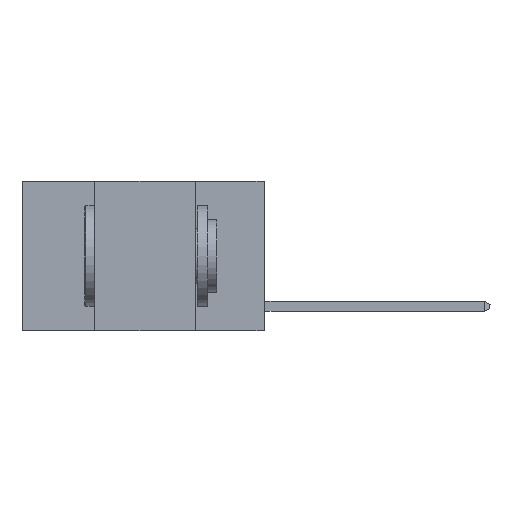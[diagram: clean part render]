
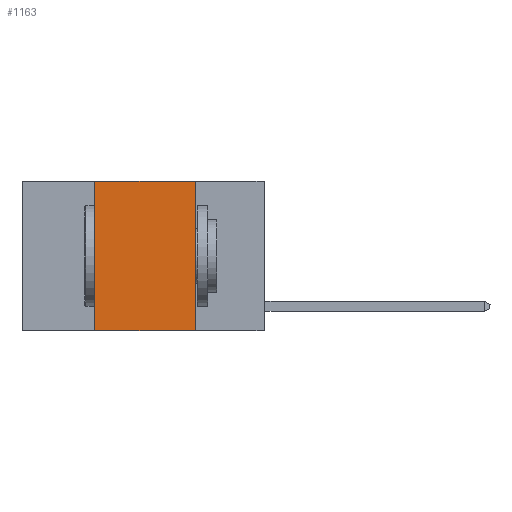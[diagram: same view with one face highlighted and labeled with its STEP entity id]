
A CAD part, left-side view. The second image highlights one B-rep face of the part: STEP entity #1163.
In plain terms, the highlighted planar face has unit normal (-1, 0, 0).
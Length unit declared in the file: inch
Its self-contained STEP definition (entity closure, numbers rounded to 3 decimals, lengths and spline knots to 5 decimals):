
#803 = AXIS2_PLACEMENT_3D ( 'NONE', #20687, #20615, #20594 ) ;
#919 = VECTOR ( 'NONE', #1184, 39.37008 ) ;
#1163 = ADVANCED_FACE ( 'NONE', ( #16370 ), #20751, .F. ) ;
#1184 = DIRECTION ( 'NONE',  ( 0., 0., -1. ) ) ;
#1397 = DIRECTION ( 'NONE',  ( 0., -1., 0. ) ) ;
#2119 = VECTOR ( 'NONE', #8049, 39.37008 ) ;
#2162 = VERTEX_POINT ( 'NONE', #7935 ) ;
#2208 = EDGE_CURVE ( 'NONE', #5200, #10174, #12425, .T. ) ;
#2625 = VERTEX_POINT ( 'NONE', #4429 ) ;
#3627 = CARTESIAN_POINT ( 'NONE',  ( 0., 0.42, -0.37 ) ) ;
#4429 = CARTESIAN_POINT ( 'NONE',  ( 0., 0.17, 0. ) ) ;
#4732 = EDGE_CURVE ( 'NONE', #2162, #2625, #10498, .T. ) ;
#5200 = VERTEX_POINT ( 'NONE', #3627 ) ;
#5351 = LINE ( 'NONE', #7872, #919 ) ;
#5489 = CARTESIAN_POINT ( 'NONE',  ( 0., 0.17, -0.37 ) ) ;
#6424 = LINE ( 'NONE', #11369, #10901 ) ;
#7872 = CARTESIAN_POINT ( 'NONE',  ( 0., 0.17, 0. ) ) ;
#7935 = CARTESIAN_POINT ( 'NONE',  ( 0., 0.42, 0. ) ) ;
#8049 = DIRECTION ( 'NONE',  ( 0., -1., 0. ) ) ;
#9613 = ORIENTED_EDGE ( 'NONE', *, *, #18906, .F. ) ;
#10137 = ORIENTED_EDGE ( 'NONE', *, *, #11545, .F. ) ;
#10174 = VERTEX_POINT ( 'NONE', #5489 ) ;
#10498 = LINE ( 'NONE', #16330, #2119 ) ;
#10901 = VECTOR ( 'NONE', #21256, 39.37008 ) ;
#11369 = CARTESIAN_POINT ( 'NONE',  ( 0., 0.42, 0. ) ) ;
#11545 = EDGE_CURVE ( 'NONE', #5200, #2162, #6424, .T. ) ;
#12425 = LINE ( 'NONE', #14746, #20735 ) ;
#14046 = ORIENTED_EDGE ( 'NONE', *, *, #4732, .F. ) ;
#14746 = CARTESIAN_POINT ( 'NONE',  ( 0., 0.6, -0.37 ) ) ;
#16330 = CARTESIAN_POINT ( 'NONE',  ( 0., 0.6, 0. ) ) ;
#16370 = FACE_OUTER_BOUND ( 'NONE', #21129, .T. ) ;
#18906 = EDGE_CURVE ( 'NONE', #2625, #10174, #5351, .T. ) ;
#18997 = ORIENTED_EDGE ( 'NONE', *, *, #2208, .T. ) ;
#20594 = DIRECTION ( 'NONE',  ( 0., 0., -1. ) ) ;
#20615 = DIRECTION ( 'NONE',  ( 1., 0., 0. ) ) ;
#20687 = CARTESIAN_POINT ( 'NONE',  ( 0., 0.6, 0. ) ) ;
#20735 = VECTOR ( 'NONE', #1397, 39.37008 ) ;
#20751 = PLANE ( 'NONE',  #803 ) ;
#21129 = EDGE_LOOP ( 'NONE', ( #9613, #14046, #10137, #18997 ) ) ;
#21256 = DIRECTION ( 'NONE',  ( 0., 0., 1. ) ) ;
